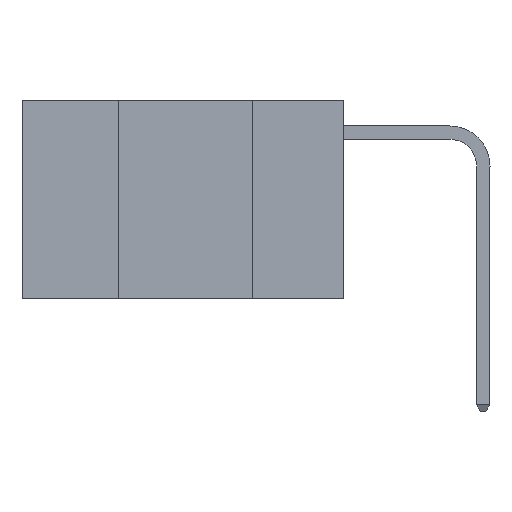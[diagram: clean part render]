
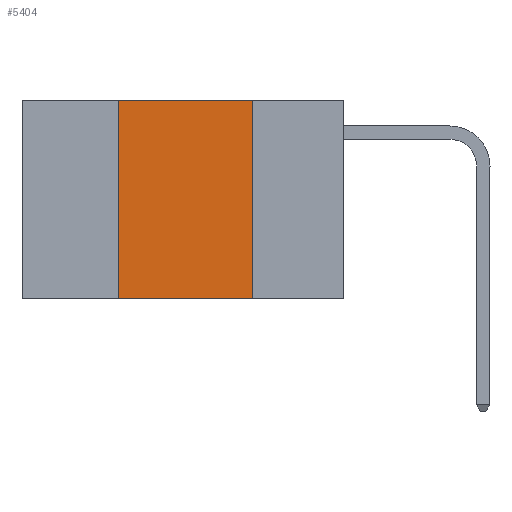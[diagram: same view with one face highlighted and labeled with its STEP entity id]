
A CAD part, left-side view. The second image highlights one B-rep face of the part: STEP entity #5404.
In plain terms, the highlighted planar face has unit normal (-1, 0, 0).
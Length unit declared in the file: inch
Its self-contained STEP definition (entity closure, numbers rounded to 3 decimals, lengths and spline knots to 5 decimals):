
#77 = LINE ( 'NONE', #11548, #2661 ) ;
#97 = CARTESIAN_POINT ( 'NONE',  ( 0., 0.6, 0. ) ) ;
#152 = DIRECTION ( 'NONE',  ( 0., -1., 0. ) ) ;
#540 = VECTOR ( 'NONE', #11680, 39.37008 ) ;
#549 = FACE_OUTER_BOUND ( 'NONE', #8390, .T. ) ;
#793 = DIRECTION ( 'NONE',  ( 0., 0., 1. ) ) ;
#1233 = AXIS2_PLACEMENT_3D ( 'NONE', #1242, #11901, #5791 ) ;
#1242 = CARTESIAN_POINT ( 'NONE',  ( 0., 0.6, 0. ) ) ;
#2033 = CARTESIAN_POINT ( 'NONE',  ( 0., 0.6, -0.37 ) ) ;
#2279 = PLANE ( 'NONE',  #1233 ) ;
#2327 = VECTOR ( 'NONE', #152, 39.37008 ) ;
#2661 = VECTOR ( 'NONE', #12459, 39.37008 ) ;
#3253 = VERTEX_POINT ( 'NONE', #5354 ) ;
#3277 = VERTEX_POINT ( 'NONE', #7992 ) ;
#3430 = LINE ( 'NONE', #2033, #540 ) ;
#5354 = CARTESIAN_POINT ( 'NONE',  ( 0., 0.17, -0.37 ) ) ;
#5404 = ADVANCED_FACE ( 'NONE', ( #549 ), #2279, .F. ) ;
#5783 = CARTESIAN_POINT ( 'NONE',  ( 0., 0.42, -0.37 ) ) ;
#5791 = DIRECTION ( 'NONE',  ( 0., 0., -1. ) ) ;
#6469 = ORIENTED_EDGE ( 'NONE', *, *, #11896, .F. ) ;
#6757 = LINE ( 'NONE', #13346, #7507 ) ;
#7507 = VECTOR ( 'NONE', #793, 39.37008 ) ;
#7968 = CARTESIAN_POINT ( 'NONE',  ( 0., 0.17, 0. ) ) ;
#7992 = CARTESIAN_POINT ( 'NONE',  ( 0., 0.42, 0. ) ) ;
#8074 = ORIENTED_EDGE ( 'NONE', *, *, #12571, .F. ) ;
#8390 = EDGE_LOOP ( 'NONE', ( #8074, #6469, #11210, #10233 ) ) ;
#9520 = EDGE_CURVE ( 'NONE', #10911, #3253, #3430, .T. ) ;
#9596 = VERTEX_POINT ( 'NONE', #7968 ) ;
#10233 = ORIENTED_EDGE ( 'NONE', *, *, #9520, .T. ) ;
#10911 = VERTEX_POINT ( 'NONE', #5783 ) ;
#11210 = ORIENTED_EDGE ( 'NONE', *, *, #11361, .F. ) ;
#11302 = LINE ( 'NONE', #97, #2327 ) ;
#11361 = EDGE_CURVE ( 'NONE', #10911, #3277, #6757, .T. ) ;
#11548 = CARTESIAN_POINT ( 'NONE',  ( 0., 0.17, 0. ) ) ;
#11680 = DIRECTION ( 'NONE',  ( 0., -1., 0. ) ) ;
#11896 = EDGE_CURVE ( 'NONE', #3277, #9596, #11302, .T. ) ;
#11901 = DIRECTION ( 'NONE',  ( 1., 0., 0. ) ) ;
#12459 = DIRECTION ( 'NONE',  ( 0., 0., -1. ) ) ;
#12571 = EDGE_CURVE ( 'NONE', #9596, #3253, #77, .T. ) ;
#13346 = CARTESIAN_POINT ( 'NONE',  ( 0., 0.42, 0. ) ) ;
